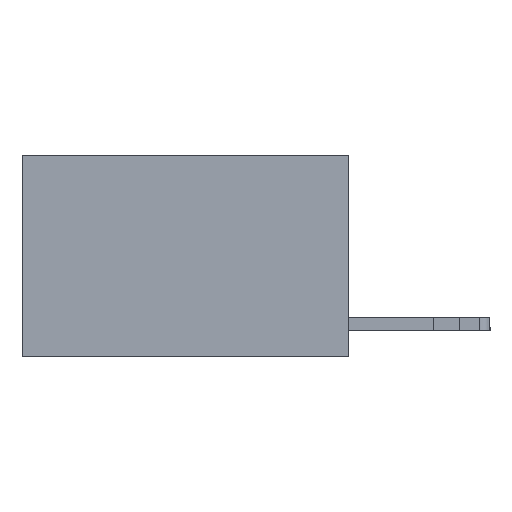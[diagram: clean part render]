
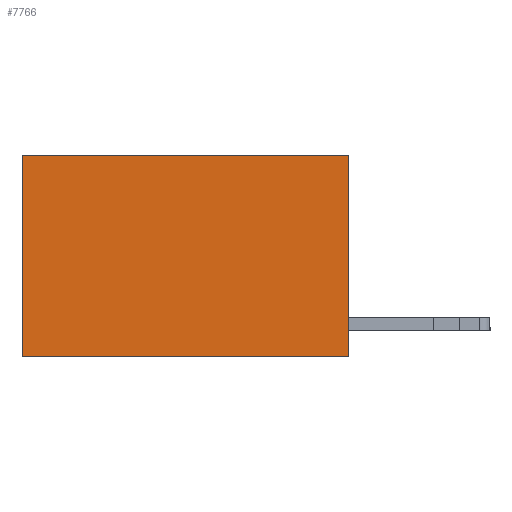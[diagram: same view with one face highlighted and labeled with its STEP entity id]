
A CAD part, left-side view. The second image highlights one B-rep face of the part: STEP entity #7766.
In plain terms, the highlighted planar face has unit normal (-1, 0, 0).
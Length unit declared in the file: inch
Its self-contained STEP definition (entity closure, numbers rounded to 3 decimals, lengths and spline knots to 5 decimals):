
#1135 = DIRECTION ( 'NONE',  ( 0., 1., 0. ) ) ;
#1482 = LINE ( 'NONE', #6783, #3484 ) ;
#2072 = VECTOR ( 'NONE', #7534, 39.37008 ) ;
#2517 = LINE ( 'NONE', #4434, #13325 ) ;
#3072 = ORIENTED_EDGE ( 'NONE', *, *, #12211, .T. ) ;
#3484 = VECTOR ( 'NONE', #4644, 39.37008 ) ;
#4159 = ORIENTED_EDGE ( 'NONE', *, *, #9559, .F. ) ;
#4434 = CARTESIAN_POINT ( 'NONE',  ( 0.2625, 0., 0. ) ) ;
#4644 = DIRECTION ( 'NONE',  ( 0., 1., 0. ) ) ;
#4670 = DIRECTION ( 'NONE',  ( 0., 0., -1. ) ) ;
#4771 = EDGE_LOOP ( 'NONE', ( #13550, #8604, #4159, #3072 ) ) ;
#4870 = FACE_OUTER_BOUND ( 'NONE', #4771, .T. ) ;
#4916 = CARTESIAN_POINT ( 'NONE',  ( 0.2625, 0., 0. ) ) ;
#5109 = EDGE_CURVE ( 'NONE', #11462, #5120, #1482, .T. ) ;
#5120 = VERTEX_POINT ( 'NONE', #8860 ) ;
#5316 = LINE ( 'NONE', #11816, #2072 ) ;
#6184 = VERTEX_POINT ( 'NONE', #8195 ) ;
#6783 = CARTESIAN_POINT ( 'NONE',  ( 0.2625, 0., -0.37 ) ) ;
#7049 = AXIS2_PLACEMENT_3D ( 'NONE', #10180, #8122, #4670 ) ;
#7161 = EDGE_CURVE ( 'NONE', #8464, #5120, #5316, .T. ) ;
#7534 = DIRECTION ( 'NONE',  ( 0., 0., -1. ) ) ;
#7766 = ADVANCED_FACE ( 'NONE', ( #4870 ), #11216, .F. ) ;
#8122 = DIRECTION ( 'NONE',  ( 1., 0., 0. ) ) ;
#8195 = CARTESIAN_POINT ( 'NONE',  ( 0.2625, 0., 0. ) ) ;
#8464 = VERTEX_POINT ( 'NONE', #12826 ) ;
#8604 = ORIENTED_EDGE ( 'NONE', *, *, #5109, .F. ) ;
#8860 = CARTESIAN_POINT ( 'NONE',  ( 0.2625, 0.6, -0.37 ) ) ;
#9071 = LINE ( 'NONE', #4916, #9334 ) ;
#9132 = DIRECTION ( 'NONE',  ( 0., 0., -1. ) ) ;
#9334 = VECTOR ( 'NONE', #9132, 39.37008 ) ;
#9559 = EDGE_CURVE ( 'NONE', #6184, #11462, #9071, .T. ) ;
#9974 = CARTESIAN_POINT ( 'NONE',  ( 0.2625, 0., -0.37 ) ) ;
#10180 = CARTESIAN_POINT ( 'NONE',  ( 0.2625, 0., 0. ) ) ;
#11216 = PLANE ( 'NONE',  #7049 ) ;
#11462 = VERTEX_POINT ( 'NONE', #9974 ) ;
#11816 = CARTESIAN_POINT ( 'NONE',  ( 0.2625, 0.6, 0. ) ) ;
#12211 = EDGE_CURVE ( 'NONE', #6184, #8464, #2517, .T. ) ;
#12826 = CARTESIAN_POINT ( 'NONE',  ( 0.2625, 0.6, 0. ) ) ;
#13325 = VECTOR ( 'NONE', #1135, 39.37008 ) ;
#13550 = ORIENTED_EDGE ( 'NONE', *, *, #7161, .T. ) ;
